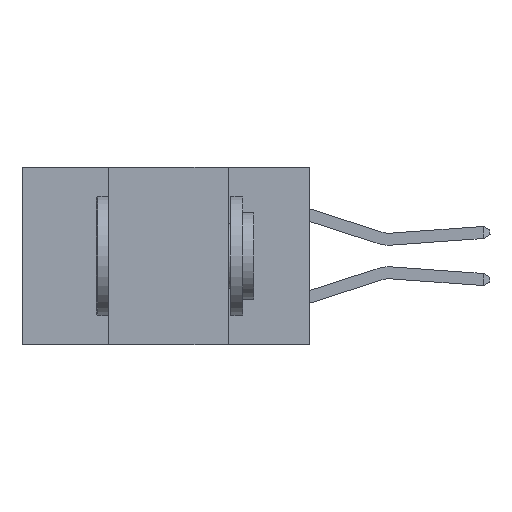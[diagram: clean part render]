
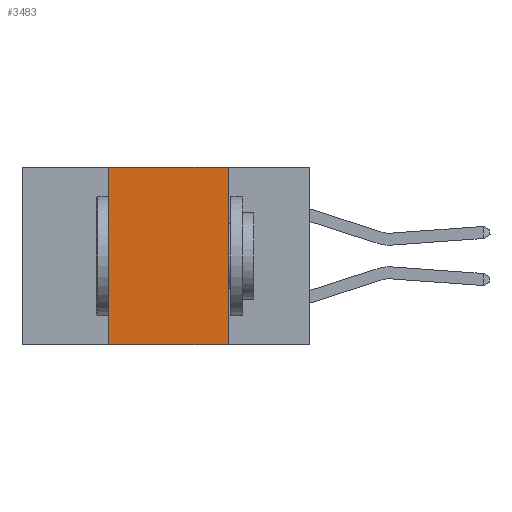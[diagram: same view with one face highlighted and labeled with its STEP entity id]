
A CAD part, left-side view. The second image highlights one B-rep face of the part: STEP entity #3483.
In plain terms, the highlighted planar face has unit normal (-1, 0, 0).
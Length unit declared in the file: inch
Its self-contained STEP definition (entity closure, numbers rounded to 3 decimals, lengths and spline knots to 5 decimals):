
#423 = CARTESIAN_POINT ( 'NONE',  ( 0., 0.6, 0. ) ) ;
#903 = ORIENTED_EDGE ( 'NONE', *, *, #13885, .F. ) ;
#1446 = VECTOR ( 'NONE', #12762, 39.37008 ) ;
#2342 = CARTESIAN_POINT ( 'NONE',  ( 0., 0.17, 0. ) ) ;
#2381 = CARTESIAN_POINT ( 'NONE',  ( 0., 0.17, -0.37 ) ) ;
#2699 = EDGE_CURVE ( 'NONE', #17308, #9035, #12845, .T. ) ;
#2987 = ORIENTED_EDGE ( 'NONE', *, *, #2699, .T. ) ;
#3438 = VECTOR ( 'NONE', #3449, 39.37008 ) ;
#3449 = DIRECTION ( 'NONE',  ( 0., 0., -1. ) ) ;
#3483 = ADVANCED_FACE ( 'NONE', ( #13652 ), #13104, .F. ) ;
#3646 = CARTESIAN_POINT ( 'NONE',  ( 0., 0.42, -0.37 ) ) ;
#4962 = LINE ( 'NONE', #423, #14343 ) ;
#5287 = EDGE_CURVE ( 'NONE', #8368, #9035, #12783, .T. ) ;
#7417 = VECTOR ( 'NONE', #15505, 39.37008 ) ;
#8368 = VERTEX_POINT ( 'NONE', #15494 ) ;
#8582 = EDGE_CURVE ( 'NONE', #17308, #17129, #15411, .T. ) ;
#8690 = CARTESIAN_POINT ( 'NONE',  ( 0., 0.6, -0.37 ) ) ;
#9035 = VERTEX_POINT ( 'NONE', #2381 ) ;
#9280 = CARTESIAN_POINT ( 'NONE',  ( 0., 0.42, 0. ) ) ;
#11249 = CARTESIAN_POINT ( 'NONE',  ( 0., 0.42, 0. ) ) ;
#11846 = DIRECTION ( 'NONE',  ( 1., 0., 0. ) ) ;
#11935 = EDGE_LOOP ( 'NONE', ( #14104, #903, #17069, #2987 ) ) ;
#12762 = DIRECTION ( 'NONE',  ( 0., 0., 1. ) ) ;
#12783 = LINE ( 'NONE', #2342, #3438 ) ;
#12845 = LINE ( 'NONE', #8690, #7417 ) ;
#13005 = DIRECTION ( 'NONE',  ( 0., 0., -1. ) ) ;
#13104 = PLANE ( 'NONE',  #14526 ) ;
#13652 = FACE_OUTER_BOUND ( 'NONE', #11935, .T. ) ;
#13885 = EDGE_CURVE ( 'NONE', #17129, #8368, #4962, .T. ) ;
#14104 = ORIENTED_EDGE ( 'NONE', *, *, #5287, .F. ) ;
#14343 = VECTOR ( 'NONE', #16609, 39.37008 ) ;
#14398 = CARTESIAN_POINT ( 'NONE',  ( 0., 0.6, 0. ) ) ;
#14526 = AXIS2_PLACEMENT_3D ( 'NONE', #14398, #11846, #13005 ) ;
#15411 = LINE ( 'NONE', #11249, #1446 ) ;
#15494 = CARTESIAN_POINT ( 'NONE',  ( 0., 0.17, 0. ) ) ;
#15505 = DIRECTION ( 'NONE',  ( 0., -1., 0. ) ) ;
#16609 = DIRECTION ( 'NONE',  ( 0., -1., 0. ) ) ;
#17069 = ORIENTED_EDGE ( 'NONE', *, *, #8582, .F. ) ;
#17129 = VERTEX_POINT ( 'NONE', #9280 ) ;
#17308 = VERTEX_POINT ( 'NONE', #3646 ) ;
